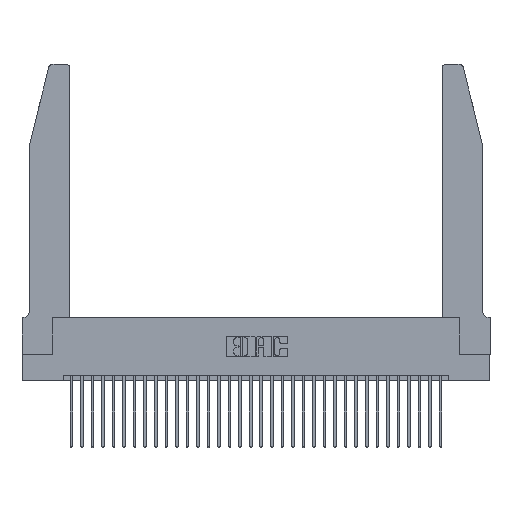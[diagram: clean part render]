
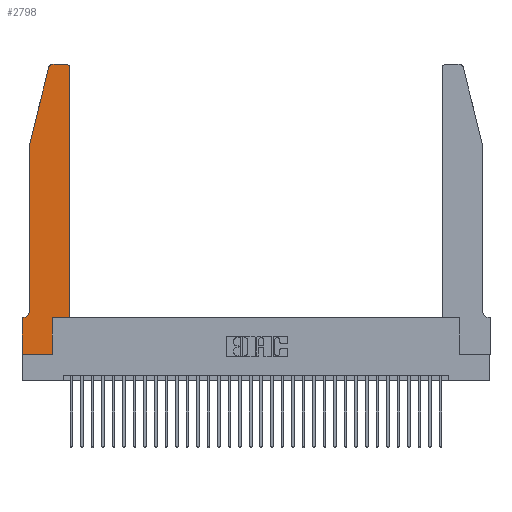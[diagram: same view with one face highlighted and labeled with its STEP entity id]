
A CAD part, top view. The second image highlights one B-rep face of the part: STEP entity #2798.
In plain terms, the highlighted planar face has unit normal (0, 0, 1).
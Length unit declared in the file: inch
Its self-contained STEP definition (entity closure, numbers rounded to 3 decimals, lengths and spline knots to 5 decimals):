
#11 = VERTEX_POINT ( 'NONE', #10491 ) ;
#354 = CARTESIAN_POINT ( 'NONE',  ( 0.25487, 2.72718, 0.37 ) ) ;
#357 = ORIENTED_EDGE ( 'NONE', *, *, #26890, .T. ) ;
#1060 = VECTOR ( 'NONE', #13269, 39.37008 ) ;
#1111 = AXIS2_PLACEMENT_3D ( 'NONE', #18666, #2724, #21243 ) ;
#1479 = ORIENTED_EDGE ( 'NONE', *, *, #21381, .T. ) ;
#1503 = ORIENTED_EDGE ( 'NONE', *, *, #18216, .T. ) ;
#1834 = CARTESIAN_POINT ( 'NONE',  ( 0.2605, 2.75, 0.37 ) ) ;
#1847 = LINE ( 'NONE', #25923, #8167 ) ;
#1912 = EDGE_CURVE ( 'NONE', #11, #11450, #8517, .T. ) ;
#2394 = CARTESIAN_POINT ( 'NONE',  ( 0.284, 2.75, 0.37 ) ) ;
#2462 = CARTESIAN_POINT ( 'NONE',  ( 0., 0., 0.37 ) ) ;
#2724 = DIRECTION ( 'NONE',  ( 0., 0., -1. ) ) ;
#2798 = ADVANCED_FACE ( 'NONE', ( #23142 ), #6250, .T. ) ;
#2822 = CARTESIAN_POINT ( 'NONE',  ( 0.2865, 0.35, 0.37 ) ) ;
#2849 = LINE ( 'NONE', #6906, #10843 ) ;
#2883 = EDGE_CURVE ( 'NONE', #31823, #11, #27539, .T. ) ;
#3039 = VECTOR ( 'NONE', #23229, 39.37008 ) ;
#3117 = EDGE_CURVE ( 'NONE', #29733, #15571, #21148, .T. ) ;
#3299 = AXIS2_PLACEMENT_3D ( 'NONE', #25796, #10270, #28357 ) ;
#3901 = LINE ( 'NONE', #4864, #3039 ) ;
#4002 = ORIENTED_EDGE ( 'NONE', *, *, #2883, .T. ) ;
#4038 = ORIENTED_EDGE ( 'NONE', *, *, #6387, .T. ) ;
#4140 = CIRCLE ( 'NONE', #17616, 0.03 ) ;
#4864 = CARTESIAN_POINT ( 'NONE',  ( 0.2865, 0.35, 0.37 ) ) ;
#5275 = ORIENTED_EDGE ( 'NONE', *, *, #8371, .T. ) ;
#6159 = DIRECTION ( 'NONE',  ( 0., 0., 1. ) ) ;
#6250 = PLANE ( 'NONE',  #29657 ) ;
#6387 = EDGE_CURVE ( 'NONE', #11450, #12281, #12453, .T. ) ;
#6906 = CARTESIAN_POINT ( 'NONE',  ( 0., 0., 0.37 ) ) ;
#7862 = CARTESIAN_POINT ( 'NONE',  ( 0.0755, 2., 0.37 ) ) ;
#8167 = VECTOR ( 'NONE', #15835, 39.37008 ) ;
#8219 = LINE ( 'NONE', #2462, #1060 ) ;
#8234 = VECTOR ( 'NONE', #27628, 39.37008 ) ;
#8371 = EDGE_CURVE ( 'NONE', #32265, #9649, #3901, .T. ) ;
#8517 = CIRCLE ( 'NONE', #1111, 0.07 ) ;
#8692 = CARTESIAN_POINT ( 'NONE',  ( 0., 0.35, 0.37 ) ) ;
#8727 = VECTOR ( 'NONE', #28897, 39.37008 ) ;
#8914 = ORIENTED_EDGE ( 'NONE', *, *, #19538, .T. ) ;
#8952 = DIRECTION ( 'NONE',  ( 1., 0., 0. ) ) ;
#9021 = CARTESIAN_POINT ( 'NONE',  ( 0.4505, 0.35, 0.37 ) ) ;
#9588 = DIRECTION ( 'NONE',  ( 1., 0., 0. ) ) ;
#9649 = VERTEX_POINT ( 'NONE', #2822 ) ;
#9692 = VERTEX_POINT ( 'NONE', #354 ) ;
#9934 = CARTESIAN_POINT ( 'NONE',  ( 0.4205, 2.75, 0.37 ) ) ;
#10270 = DIRECTION ( 'NONE',  ( 0., 0., 1. ) ) ;
#10491 = CARTESIAN_POINT ( 'NONE',  ( 0.0755, 0.42, 0.37 ) ) ;
#10829 = CARTESIAN_POINT ( 'NONE',  ( 0.0755, 2., 0.37 ) ) ;
#10843 = VECTOR ( 'NONE', #9588, 39.37008 ) ;
#11128 = CIRCLE ( 'NONE', #3299, 0.03 ) ;
#11450 = VERTEX_POINT ( 'NONE', #18285 ) ;
#11602 = EDGE_CURVE ( 'NONE', #15571, #9692, #4140, .T. ) ;
#11614 = VECTOR ( 'NONE', #14226, 39.37008 ) ;
#12281 = VERTEX_POINT ( 'NONE', #8692 ) ;
#12453 = LINE ( 'NONE', #22000, #11614 ) ;
#12867 = ORIENTED_EDGE ( 'NONE', *, *, #29878, .T. ) ;
#13269 = DIRECTION ( 'NONE',  ( 0., -1., 0. ) ) ;
#14226 = DIRECTION ( 'NONE',  ( -1., 0., 0. ) ) ;
#14296 = VECTOR ( 'NONE', #15296, 39.37008 ) ;
#14533 = CARTESIAN_POINT ( 'NONE',  ( 0.0755, 2., 0.37 ) ) ;
#15296 = DIRECTION ( 'NONE',  ( -1., 0., 0. ) ) ;
#15571 = VERTEX_POINT ( 'NONE', #2394 ) ;
#15835 = DIRECTION ( 'NONE',  ( 0., 1., 0. ) ) ;
#15908 = CARTESIAN_POINT ( 'NONE',  ( 0.4505, 2.72, 0.37 ) ) ;
#16129 = LINE ( 'NONE', #25053, #8234 ) ;
#16434 = ORIENTED_EDGE ( 'NONE', *, *, #32236, .T. ) ;
#17616 = AXIS2_PLACEMENT_3D ( 'NONE', #21889, #6159, #24444 ) ;
#18116 = ORIENTED_EDGE ( 'NONE', *, *, #1912, .T. ) ;
#18216 = EDGE_CURVE ( 'NONE', #9692, #31823, #22591, .T. ) ;
#18285 = CARTESIAN_POINT ( 'NONE',  ( 0.0055, 0.35, 0.37 ) ) ;
#18666 = CARTESIAN_POINT ( 'NONE',  ( 0.0055, 0.42, 0.37 ) ) ;
#19538 = EDGE_CURVE ( 'NONE', #20175, #29733, #11128, .T. ) ;
#20175 = VERTEX_POINT ( 'NONE', #15908 ) ;
#20620 = CARTESIAN_POINT ( 'NONE',  ( 0., 0., 0.37 ) ) ;
#20774 = VECTOR ( 'NONE', #32462, 39.37008 ) ;
#21148 = LINE ( 'NONE', #1834, #14296 ) ;
#21243 = DIRECTION ( 'NONE',  ( -1., 0., 0. ) ) ;
#21381 = EDGE_CURVE ( 'NONE', #12281, #33610, #8219, .T. ) ;
#21889 = CARTESIAN_POINT ( 'NONE',  ( 0.284, 2.72, 0.37 ) ) ;
#21970 = CARTESIAN_POINT ( 'NONE',  ( 0., 0.35, 0.37 ) ) ;
#22000 = CARTESIAN_POINT ( 'NONE',  ( 0.0755, 0.35, 0.37 ) ) ;
#22591 = LINE ( 'NONE', #10829, #8727 ) ;
#23142 = FACE_OUTER_BOUND ( 'NONE', #25088, .T. ) ;
#23229 = DIRECTION ( 'NONE',  ( 0., 1., 0. ) ) ;
#23360 = ORIENTED_EDGE ( 'NONE', *, *, #11602, .T. ) ;
#24444 = DIRECTION ( 'NONE',  ( 1., 0., 0. ) ) ;
#24528 = DIRECTION ( 'NONE',  ( 0., 0., 1. ) ) ;
#25053 = CARTESIAN_POINT ( 'NONE',  ( 0.4505, 0.35, 0.37 ) ) ;
#25088 = EDGE_LOOP ( 'NONE', ( #31336, #23360, #1503, #4002, #18116, #4038, #1479, #357, #5275, #16434, #12867, #8914 ) ) ;
#25163 = CARTESIAN_POINT ( 'NONE',  ( 0.2865, 0., 0.37 ) ) ;
#25796 = CARTESIAN_POINT ( 'NONE',  ( 0.4205, 2.72, 0.37 ) ) ;
#25923 = CARTESIAN_POINT ( 'NONE',  ( 0.4505, 0.35, 0.37 ) ) ;
#26890 = EDGE_CURVE ( 'NONE', #33610, #32265, #2849, .T. ) ;
#27539 = LINE ( 'NONE', #14533, #20774 ) ;
#27628 = DIRECTION ( 'NONE',  ( 1., 0., 0. ) ) ;
#28357 = DIRECTION ( 'NONE',  ( 1., 0., 0. ) ) ;
#28897 = DIRECTION ( 'NONE',  ( -0.239, -0.971, 0. ) ) ;
#29657 = AXIS2_PLACEMENT_3D ( 'NONE', #21970, #24528, #8952 ) ;
#29733 = VERTEX_POINT ( 'NONE', #9934 ) ;
#29878 = EDGE_CURVE ( 'NONE', #30167, #20175, #1847, .T. ) ;
#30167 = VERTEX_POINT ( 'NONE', #9021 ) ;
#31336 = ORIENTED_EDGE ( 'NONE', *, *, #3117, .T. ) ;
#31823 = VERTEX_POINT ( 'NONE', #7862 ) ;
#32236 = EDGE_CURVE ( 'NONE', #9649, #30167, #16129, .T. ) ;
#32265 = VERTEX_POINT ( 'NONE', #25163 ) ;
#32462 = DIRECTION ( 'NONE',  ( 0., -1., 0. ) ) ;
#33610 = VERTEX_POINT ( 'NONE', #20620 ) ;
